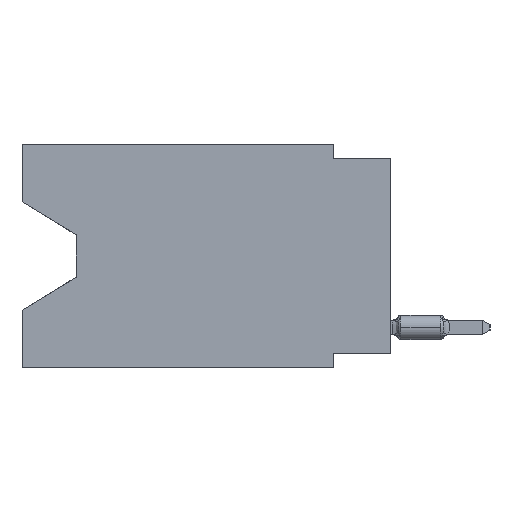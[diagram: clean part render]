
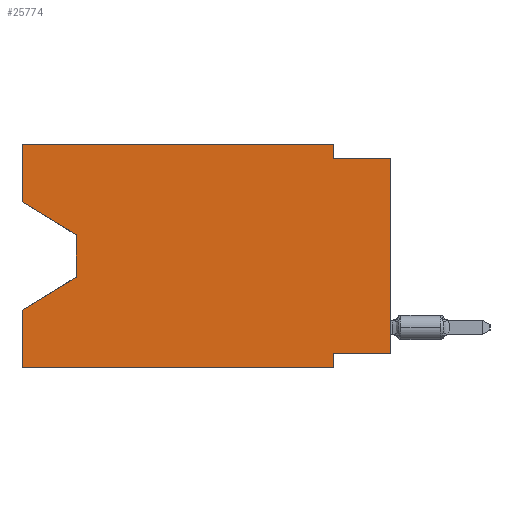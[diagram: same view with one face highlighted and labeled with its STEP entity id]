
A CAD part, left-side view. The second image highlights one B-rep face of the part: STEP entity #25774.
In plain terms, the highlighted planar face has unit normal (-1, 0, 0).
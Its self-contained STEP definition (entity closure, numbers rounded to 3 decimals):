
#79 = EDGE_CURVE ( 'NONE', #26355, #1816, #51329, .T. ) ;
#1120 = ORIENTED_EDGE ( 'NONE', *, *, #23081, .T. ) ;
#1262 = LINE ( 'NONE', #49040, #18671 ) ;
#1816 = VERTEX_POINT ( 'NONE', #63155 ) ;
#2416 = VERTEX_POINT ( 'NONE', #22261 ) ;
#2534 = VECTOR ( 'NONE', #46121, 1000. ) ;
#2665 = CARTESIAN_POINT ( 'NONE',  ( 0., 16.383, -2.546 ) ) ;
#2856 = EDGE_CURVE ( 'NONE', #51542, #64476, #40875, .T. ) ;
#3044 = ORIENTED_EDGE ( 'NONE', *, *, #2856, .T. ) ;
#3259 = LINE ( 'NONE', #9157, #62577 ) ;
#4769 = CARTESIAN_POINT ( 'NONE',  ( 0., 16.383, 0. ) ) ;
#5110 = FACE_OUTER_BOUND ( 'NONE', #58588, .T. ) ;
#5452 = PLANE ( 'NONE',  #52390 ) ;
#6189 = ORIENTED_EDGE ( 'NONE', *, *, #8161, .F. ) ;
#6496 = LINE ( 'NONE', #60175, #12006 ) ;
#6716 = CARTESIAN_POINT ( 'NONE',  ( 0., 2.54, -9.906 ) ) ;
#7907 = VERTEX_POINT ( 'NONE', #63301 ) ;
#8161 = EDGE_CURVE ( 'NONE', #60319, #25704, #66424, .T. ) ;
#8191 = CARTESIAN_POINT ( 'NONE',  ( 0., 2.54, 0. ) ) ;
#8431 = LINE ( 'NONE', #67000, #11079 ) ;
#9157 = CARTESIAN_POINT ( 'NONE',  ( 0., 13.97, -5.893 ) ) ;
#9502 = DIRECTION ( 'NONE',  ( 0., 0., -1. ) ) ;
#11079 = VECTOR ( 'NONE', #19223, 1000. ) ;
#11087 = CARTESIAN_POINT ( 'NONE',  ( 0., 0., -9.271 ) ) ;
#12006 = VECTOR ( 'NONE', #65760, 1000. ) ;
#12366 = ORIENTED_EDGE ( 'NONE', *, *, #47613, .F. ) ;
#14044 = LINE ( 'NONE', #24503, #62628 ) ;
#14713 = VECTOR ( 'NONE', #19338, 1000. ) ;
#14820 = VECTOR ( 'NONE', #64617, 1000. ) ;
#15649 = CARTESIAN_POINT ( 'NONE',  ( 0., 2.54, 0. ) ) ;
#17371 = CARTESIAN_POINT ( 'NONE',  ( 0., 16.383, -9.906 ) ) ;
#18671 = VECTOR ( 'NONE', #27061, 1000. ) ;
#19223 = DIRECTION ( 'NONE',  ( 0., -1., 0. ) ) ;
#19338 = DIRECTION ( 'NONE',  ( 0., 0., -1. ) ) ;
#21658 = CARTESIAN_POINT ( 'NONE',  ( 0., 13.97, -5.893 ) ) ;
#22261 = CARTESIAN_POINT ( 'NONE',  ( 0., 2.54, -9.271 ) ) ;
#22277 = CARTESIAN_POINT ( 'NONE',  ( 0., 2.54, -9.906 ) ) ;
#23081 = EDGE_CURVE ( 'NONE', #66744, #51542, #14044, .T. ) ;
#23114 = EDGE_CURVE ( 'NONE', #66744, #53662, #40202, .T. ) ;
#24223 = CARTESIAN_POINT ( 'NONE',  ( 0., 0., -0.635 ) ) ;
#24503 = CARTESIAN_POINT ( 'NONE',  ( 0., 16.383, -2.546 ) ) ;
#25704 = VERTEX_POINT ( 'NONE', #41019 ) ;
#25774 = ADVANCED_FACE ( 'NONE', ( #5110 ), #5452, .F. ) ;
#25907 = ORIENTED_EDGE ( 'NONE', *, *, #79, .F. ) ;
#26355 = VERTEX_POINT ( 'NONE', #17371 ) ;
#27061 = DIRECTION ( 'NONE',  ( 0., 0., 1. ) ) ;
#27595 = VERTEX_POINT ( 'NONE', #24223 ) ;
#27851 = ORIENTED_EDGE ( 'NONE', *, *, #31638, .F. ) ;
#27899 = EDGE_CURVE ( 'NONE', #53662, #60319, #63918, .T. ) ;
#28196 = DIRECTION ( 'NONE',  ( 0., 0., -1. ) ) ;
#28407 = VECTOR ( 'NONE', #67048, 1000. ) ;
#29160 = VERTEX_POINT ( 'NONE', #6716 ) ;
#31638 = EDGE_CURVE ( 'NONE', #7907, #2416, #52240, .T. ) ;
#32531 = CARTESIAN_POINT ( 'NONE',  ( 0., 16.383, 0. ) ) ;
#38248 = ORIENTED_EDGE ( 'NONE', *, *, #27899, .F. ) ;
#38552 = EDGE_CURVE ( 'NONE', #2416, #29160, #54013, .T. ) ;
#40202 = LINE ( 'NONE', #41567, #2534 ) ;
#40400 = VECTOR ( 'NONE', #28196, 1000. ) ;
#40540 = CARTESIAN_POINT ( 'NONE',  ( 0., 13.97, -4.013 ) ) ;
#40875 = LINE ( 'NONE', #40540, #51064 ) ;
#41019 = CARTESIAN_POINT ( 'NONE',  ( 0., 2.54, -0.635 ) ) ;
#41567 = CARTESIAN_POINT ( 'NONE',  ( 0., 16.383, 0. ) ) ;
#44621 = ORIENTED_EDGE ( 'NONE', *, *, #38552, .F. ) ;
#45202 = ORIENTED_EDGE ( 'NONE', *, *, #58516, .T. ) ;
#46121 = DIRECTION ( 'NONE',  ( 0., 0., 1. ) ) ;
#46761 = ORIENTED_EDGE ( 'NONE', *, *, #23114, .F. ) ;
#47613 = EDGE_CURVE ( 'NONE', #25704, #27595, #8431, .T. ) ;
#48385 = ORIENTED_EDGE ( 'NONE', *, *, #58492, .T. ) ;
#49040 = CARTESIAN_POINT ( 'NONE',  ( 0., 0., 0. ) ) ;
#50472 = EDGE_CURVE ( 'NONE', #64476, #1816, #3259, .T. ) ;
#51010 = DIRECTION ( 'NONE',  ( 0., 0.855, -0.519 ) ) ;
#51064 = VECTOR ( 'NONE', #9502, 1000. ) ;
#51329 = LINE ( 'NONE', #61106, #28407 ) ;
#51542 = VERTEX_POINT ( 'NONE', #61819 ) ;
#52240 = LINE ( 'NONE', #11087, #60705 ) ;
#52390 = AXIS2_PLACEMENT_3D ( 'NONE', #4769, #68893, #63315 ) ;
#53662 = VERTEX_POINT ( 'NONE', #59757 ) ;
#54013 = LINE ( 'NONE', #22277, #40400 ) ;
#57597 = DIRECTION ( 'NONE',  ( 0., -0.855, -0.519 ) ) ;
#58492 = EDGE_CURVE ( 'NONE', #26355, #29160, #6496, .T. ) ;
#58516 = EDGE_CURVE ( 'NONE', #7907, #27595, #1262, .T. ) ;
#58588 = EDGE_LOOP ( 'NONE', ( #1120, #3044, #59938, #25907, #48385, #44621, #27851, #45202, #12366, #6189, #38248, #46761 ) ) ;
#59757 = CARTESIAN_POINT ( 'NONE',  ( 0., 16.383, 0. ) ) ;
#59938 = ORIENTED_EDGE ( 'NONE', *, *, #50472, .T. ) ;
#60175 = CARTESIAN_POINT ( 'NONE',  ( 0., 16.383, -9.906 ) ) ;
#60319 = VERTEX_POINT ( 'NONE', #15649 ) ;
#60705 = VECTOR ( 'NONE', #62708, 1000. ) ;
#61106 = CARTESIAN_POINT ( 'NONE',  ( 0., 16.383, 0. ) ) ;
#61819 = CARTESIAN_POINT ( 'NONE',  ( 0., 13.97, -4.013 ) ) ;
#62577 = VECTOR ( 'NONE', #51010, 1000. ) ;
#62628 = VECTOR ( 'NONE', #57597, 1000. ) ;
#62708 = DIRECTION ( 'NONE',  ( 0., 1., 0. ) ) ;
#63155 = CARTESIAN_POINT ( 'NONE',  ( 0., 16.383, -7.36 ) ) ;
#63301 = CARTESIAN_POINT ( 'NONE',  ( 0., 0., -9.271 ) ) ;
#63315 = DIRECTION ( 'NONE',  ( 0., 0., -1. ) ) ;
#63918 = LINE ( 'NONE', #32531, #14820 ) ;
#64476 = VERTEX_POINT ( 'NONE', #21658 ) ;
#64617 = DIRECTION ( 'NONE',  ( 0., -1., 0. ) ) ;
#65760 = DIRECTION ( 'NONE',  ( 0., -1., 0. ) ) ;
#66424 = LINE ( 'NONE', #8191, #14713 ) ;
#66744 = VERTEX_POINT ( 'NONE', #2665 ) ;
#67000 = CARTESIAN_POINT ( 'NONE',  ( 0., 0., -0.635 ) ) ;
#67048 = DIRECTION ( 'NONE',  ( 0., 0., 1. ) ) ;
#68893 = DIRECTION ( 'NONE',  ( 1., 0., 0. ) ) ;
